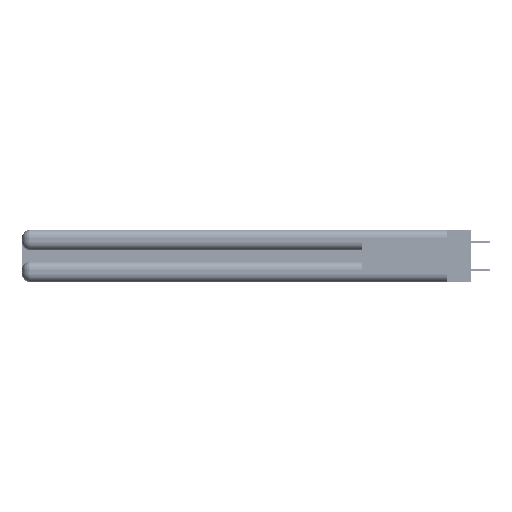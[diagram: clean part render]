
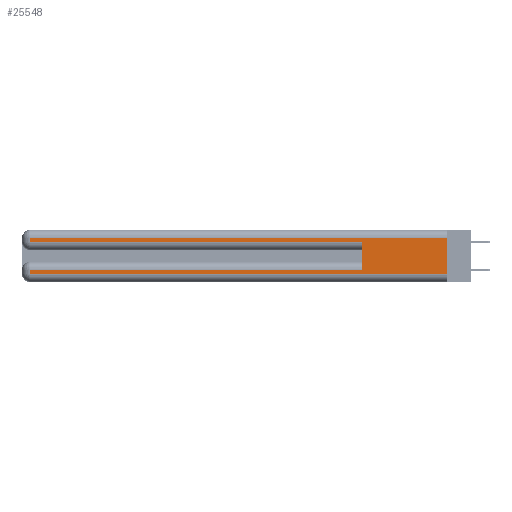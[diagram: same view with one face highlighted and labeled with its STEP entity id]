
A CAD part, left-side view. The second image highlights one B-rep face of the part: STEP entity #25548.
In plain terms, the highlighted planar face has unit normal (-1, 0, 0).
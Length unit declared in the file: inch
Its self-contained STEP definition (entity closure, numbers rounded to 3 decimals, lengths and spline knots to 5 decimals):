
#472 = DIRECTION ( 'NONE',  ( 0., 0., -1. ) ) ;
#700 = CARTESIAN_POINT ( 'NONE',  ( 0., 0., 0.31 ) ) ;
#711 = CARTESIAN_POINT ( 'NONE',  ( 0., 2.94, 0.37 ) ) ;
#3010 = LINE ( 'NONE', #36735, #40525 ) ;
#4404 = CARTESIAN_POINT ( 'NONE',  ( 0., 2.94, 0.285 ) ) ;
#4491 = EDGE_CURVE ( 'NONE', #18214, #49354, #42986, .T. ) ;
#6463 = CARTESIAN_POINT ( 'NONE',  ( 0., 2.94, 0.31 ) ) ;
#6780 = EDGE_CURVE ( 'NONE', #19300, #39359, #10669, .T. ) ;
#6830 = CARTESIAN_POINT ( 'NONE',  ( 0., 0., 0.37 ) ) ;
#8085 = EDGE_CURVE ( 'NONE', #19300, #20530, #30612, .T. ) ;
#10414 = LINE ( 'NONE', #47481, #24784 ) ;
#10669 = LINE ( 'NONE', #22316, #39099 ) ;
#10682 = VERTEX_POINT ( 'NONE', #24108 ) ;
#10700 = PLANE ( 'NONE',  #53131 ) ;
#11851 = DIRECTION ( 'NONE',  ( 0., -1., 0. ) ) ;
#12110 = LINE ( 'NONE', #29006, #29957 ) ;
#12881 = ORIENTED_EDGE ( 'NONE', *, *, #48573, .F. ) ;
#13170 = ORIENTED_EDGE ( 'NONE', *, *, #6780, .F. ) ;
#14056 = ORIENTED_EDGE ( 'NONE', *, *, #8085, .T. ) ;
#17954 = LINE ( 'NONE', #44744, #32359 ) ;
#17959 = ORIENTED_EDGE ( 'NONE', *, *, #50159, .T. ) ;
#18018 = EDGE_CURVE ( 'NONE', #20530, #10682, #30302, .T. ) ;
#18214 = VERTEX_POINT ( 'NONE', #26420 ) ;
#19056 = DIRECTION ( 'NONE',  ( 0., 0., -1. ) ) ;
#19094 = CARTESIAN_POINT ( 'NONE',  ( 0., 0.6, 0.085 ) ) ;
#19300 = VERTEX_POINT ( 'NONE', #19094 ) ;
#19428 = VERTEX_POINT ( 'NONE', #4404 ) ;
#20530 = VERTEX_POINT ( 'NONE', #54506 ) ;
#21015 = EDGE_CURVE ( 'NONE', #10682, #53648, #12110, .T. ) ;
#22316 = CARTESIAN_POINT ( 'NONE',  ( 0., 0.6, 0.145 ) ) ;
#23738 = CARTESIAN_POINT ( 'NONE',  ( 0., 0., 0.06 ) ) ;
#24108 = CARTESIAN_POINT ( 'NONE',  ( 0., 2.94, 0.06 ) ) ;
#24784 = VECTOR ( 'NONE', #39186, 39.37008 ) ;
#25071 = ORIENTED_EDGE ( 'NONE', *, *, #4491, .T. ) ;
#25548 = ADVANCED_FACE ( 'NONE', ( #40821 ), #10700, .F. ) ;
#25882 = DIRECTION ( 'NONE',  ( 0., 0., -1. ) ) ;
#26261 = CARTESIAN_POINT ( 'NONE',  ( 0., 0.6, 0.285 ) ) ;
#26420 = CARTESIAN_POINT ( 'NONE',  ( 0., 0., 0.31 ) ) ;
#29006 = CARTESIAN_POINT ( 'NONE',  ( 0., 0., 0.06 ) ) ;
#29957 = VECTOR ( 'NONE', #11851, 39.37008 ) ;
#30302 = LINE ( 'NONE', #711, #47398 ) ;
#30612 = LINE ( 'NONE', #49800, #34449 ) ;
#32359 = VECTOR ( 'NONE', #19056, 39.37008 ) ;
#34260 = EDGE_LOOP ( 'NONE', ( #12881, #25071, #43040, #17959, #13170, #14056, #50603, #54212 ) ) ;
#34449 = VECTOR ( 'NONE', #37345, 39.37008 ) ;
#35302 = DIRECTION ( 'NONE',  ( 0., 0., 1. ) ) ;
#36735 = CARTESIAN_POINT ( 'NONE',  ( 0., 0., 0.37 ) ) ;
#37345 = DIRECTION ( 'NONE',  ( 0., 1., 0. ) ) ;
#39099 = VECTOR ( 'NONE', #35302, 39.37008 ) ;
#39186 = DIRECTION ( 'NONE',  ( 0., -1., 0. ) ) ;
#39359 = VERTEX_POINT ( 'NONE', #26261 ) ;
#40525 = VECTOR ( 'NONE', #472, 39.37008 ) ;
#40821 = FACE_OUTER_BOUND ( 'NONE', #34260, .T. ) ;
#42986 = LINE ( 'NONE', #700, #47759 ) ;
#43040 = ORIENTED_EDGE ( 'NONE', *, *, #53606, .T. ) ;
#44744 = CARTESIAN_POINT ( 'NONE',  ( 0., 2.94, 0.37 ) ) ;
#45254 = DIRECTION ( 'NONE',  ( 0., 0., -1. ) ) ;
#46335 = DIRECTION ( 'NONE',  ( 0., 1., 0. ) ) ;
#47398 = VECTOR ( 'NONE', #25882, 39.37008 ) ;
#47481 = CARTESIAN_POINT ( 'NONE',  ( 0., 0., 0.285 ) ) ;
#47759 = VECTOR ( 'NONE', #46335, 39.37008 ) ;
#48573 = EDGE_CURVE ( 'NONE', #18214, #53648, #3010, .T. ) ;
#49354 = VERTEX_POINT ( 'NONE', #6463 ) ;
#49800 = CARTESIAN_POINT ( 'NONE',  ( 0., 0., 0.085 ) ) ;
#50159 = EDGE_CURVE ( 'NONE', #19428, #39359, #10414, .T. ) ;
#50603 = ORIENTED_EDGE ( 'NONE', *, *, #18018, .T. ) ;
#53018 = DIRECTION ( 'NONE',  ( 1., 0., 0. ) ) ;
#53131 = AXIS2_PLACEMENT_3D ( 'NONE', #6830, #53018, #45254 ) ;
#53606 = EDGE_CURVE ( 'NONE', #49354, #19428, #17954, .T. ) ;
#53648 = VERTEX_POINT ( 'NONE', #23738 ) ;
#54212 = ORIENTED_EDGE ( 'NONE', *, *, #21015, .T. ) ;
#54506 = CARTESIAN_POINT ( 'NONE',  ( 0., 2.94, 0.085 ) ) ;
